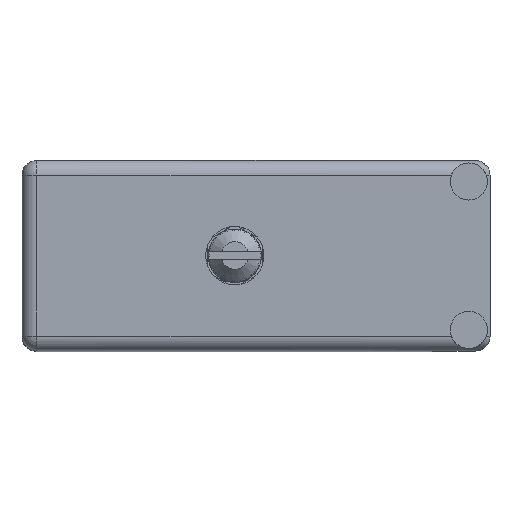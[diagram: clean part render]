
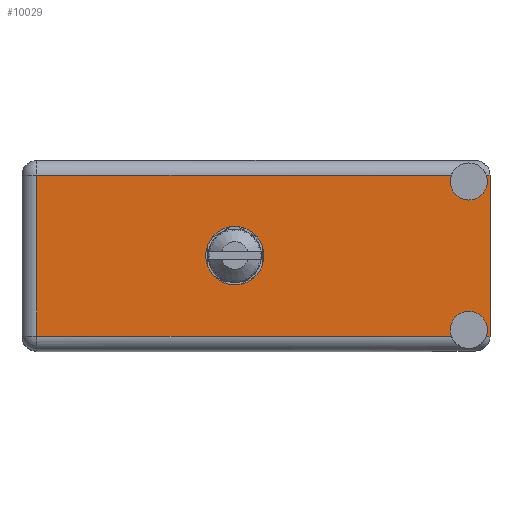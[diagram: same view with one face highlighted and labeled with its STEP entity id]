
A CAD part, top view. The second image highlights one B-rep face of the part: STEP entity #10029.
In plain terms, the highlighted face is planar.
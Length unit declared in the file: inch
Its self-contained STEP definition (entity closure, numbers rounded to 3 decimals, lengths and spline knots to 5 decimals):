
#2660 = EDGE_CURVE ( 'NONE', #68356, #49674, #86498, .T. ) ;
#3480 = DIRECTION ( 'NONE',  ( -1., 0., 0. ) ) ;
#7040 = AXIS2_PLACEMENT_3D ( 'NONE', #87515, #70118, #33771 ) ;
#8660 = ORIENTED_EDGE ( 'NONE', *, *, #97273, .F. ) ;
#10029 = ADVANCED_FACE ( 'NONE', ( #74525, #39920 ), #23921, .T. ) ;
#12254 = CARTESIAN_POINT ( 'NONE',  ( 1.204, 1.466, 0.3795 ) ) ;
#12378 = DIRECTION ( 'NONE',  ( 0., 0., 1. ) ) ;
#12601 = CARTESIAN_POINT ( 'NONE',  ( 1.18638, 1.466, 0.3795 ) ) ;
#12621 = ORIENTED_EDGE ( 'NONE', *, *, #48235, .T. ) ;
#12693 = VECTOR ( 'NONE', #94890, 39.37008 ) ;
#13507 = DIRECTION ( 'NONE',  ( 0., 1., 0. ) ) ;
#15020 = DIRECTION ( 'NONE',  ( 0., 1., 0. ) ) ;
#15229 = VECTOR ( 'NONE', #3480, 39.37008 ) ;
#16749 = ORIENTED_EDGE ( 'NONE', *, *, #27406, .F. ) ;
#18102 = CARTESIAN_POINT ( 'NONE',  ( 0., 1.466, 0. ) ) ;
#18825 = CARTESIAN_POINT ( 'NONE',  ( 1.204, 1.466, -0.3795 ) ) ;
#20325 = VECTOR ( 'NONE', #26297, 39.37008 ) ;
#23921 = PLANE ( 'NONE',  #24233 ) ;
#24233 = AXIS2_PLACEMENT_3D ( 'NONE', #24301, #15020, #112948 ) ;
#24301 = CARTESIAN_POINT ( 'NONE',  ( -1.004, 1.466, -0.4495 ) ) ;
#24703 = CIRCLE ( 'NONE', #62095, 0.1375 ) ;
#26297 = DIRECTION ( 'NONE',  ( -1., 0., 0. ) ) ;
#26575 = CARTESIAN_POINT ( 'NONE',  ( 1.104, 1.466, -0.2625 ) ) ;
#27406 = EDGE_CURVE ( 'NONE', #49674, #68356, #24703, .T. ) ;
#28528 = VECTOR ( 'NONE', #70282, 39.37008 ) ;
#30083 = AXIS2_PLACEMENT_3D ( 'NONE', #67349, #13507, #94017 ) ;
#31822 = ORIENTED_EDGE ( 'NONE', *, *, #79297, .T. ) ;
#32850 = VERTEX_POINT ( 'NONE', #46382 ) ;
#33526 = AXIS2_PLACEMENT_3D ( 'NONE', #114752, #53202, #61726 ) ;
#33771 = DIRECTION ( 'NONE',  ( 0., 0., 1. ) ) ;
#35325 = ORIENTED_EDGE ( 'NONE', *, *, #82789, .F. ) ;
#39052 = VERTEX_POINT ( 'NONE', #109235 ) ;
#39732 = CARTESIAN_POINT ( 'NONE',  ( 1.104, 1.466, 0.2625 ) ) ;
#39920 = FACE_OUTER_BOUND ( 'NONE', #98981, .T. ) ;
#40846 = VERTEX_POINT ( 'NONE', #26575 ) ;
#41012 = AXIS2_PLACEMENT_3D ( 'NONE', #105422, #43163, #105036 ) ;
#41634 = LINE ( 'NONE', #56622, #15229 ) ;
#43163 = DIRECTION ( 'NONE',  ( 0., 1., 0. ) ) ;
#43853 = CARTESIAN_POINT ( 'NONE',  ( 0., 1.466, 0.1375 ) ) ;
#44216 = EDGE_CURVE ( 'NONE', #54814, #94018, #106406, .T. ) ;
#45693 = EDGE_CURVE ( 'NONE', #59850, #95117, #46134, .T. ) ;
#46134 = CIRCLE ( 'NONE', #67799, 0.0875 ) ;
#46382 = CARTESIAN_POINT ( 'NONE',  ( 1.18638, 1.466, -0.3795 ) ) ;
#47016 = CARTESIAN_POINT ( 'NONE',  ( -0.934, 1.466, -0.3795 ) ) ;
#48092 = ORIENTED_EDGE ( 'NONE', *, *, #86106, .F. ) ;
#48235 = EDGE_CURVE ( 'NONE', #59850, #99988, #88930, .T. ) ;
#48389 = VECTOR ( 'NONE', #92002, 39.37008 ) ;
#49674 = VERTEX_POINT ( 'NONE', #92686 ) ;
#50212 = ORIENTED_EDGE ( 'NONE', *, *, #109368, .T. ) ;
#51059 = CARTESIAN_POINT ( 'NONE',  ( -0.934, 1.466, 0.3795 ) ) ;
#51062 = EDGE_CURVE ( 'NONE', #94018, #39052, #70531, .T. ) ;
#52126 = LINE ( 'NONE', #98083, #28528 ) ;
#53202 = DIRECTION ( 'NONE',  ( 0., 1., 0. ) ) ;
#54814 = VERTEX_POINT ( 'NONE', #47016 ) ;
#55426 = CIRCLE ( 'NONE', #33526, 0.0875 ) ;
#56526 = CARTESIAN_POINT ( 'NONE',  ( 1.104, 1.466, 0.35 ) ) ;
#56622 = CARTESIAN_POINT ( 'NONE',  ( -1.004, 1.466, -0.3795 ) ) ;
#56725 = VERTEX_POINT ( 'NONE', #111007 ) ;
#58659 = ORIENTED_EDGE ( 'NONE', *, *, #44216, .T. ) ;
#59850 = VERTEX_POINT ( 'NONE', #12601 ) ;
#61726 = DIRECTION ( 'NONE',  ( 0., 0., 1. ) ) ;
#61834 = ORIENTED_EDGE ( 'NONE', *, *, #2660, .F. ) ;
#61856 = DIRECTION ( 'NONE',  ( 0., 0., 1. ) ) ;
#62095 = AXIS2_PLACEMENT_3D ( 'NONE', #18102, #80007, #61856 ) ;
#64334 = VERTEX_POINT ( 'NONE', #18825 ) ;
#65453 = DIRECTION ( 'NONE',  ( 0., 1., 0. ) ) ;
#67349 = CARTESIAN_POINT ( 'NONE',  ( 1.104, 1.466, 0.35 ) ) ;
#67799 = AXIS2_PLACEMENT_3D ( 'NONE', #56526, #65453, #12378 ) ;
#68356 = VERTEX_POINT ( 'NONE', #43853 ) ;
#70118 = DIRECTION ( 'NONE',  ( 0., 1., 0. ) ) ;
#70282 = DIRECTION ( 'NONE',  ( 0., 0., 1. ) ) ;
#70531 = LINE ( 'NONE', #12254, #48389 ) ;
#71077 = ORIENTED_EDGE ( 'NONE', *, *, #90333, .F. ) ;
#71566 = CARTESIAN_POINT ( 'NONE',  ( -1.004, 1.466, -0.3795 ) ) ;
#72995 = LINE ( 'NONE', #71566, #20325 ) ;
#74092 = ORIENTED_EDGE ( 'NONE', *, *, #45693, .F. ) ;
#74525 = FACE_BOUND ( 'NONE', #97486, .T. ) ;
#79297 = EDGE_CURVE ( 'NONE', #56725, #54814, #41634, .T. ) ;
#80007 = DIRECTION ( 'NONE',  ( 0., 1., 0. ) ) ;
#82789 = EDGE_CURVE ( 'NONE', #64334, #99988, #52126, .T. ) ;
#83627 = CIRCLE ( 'NONE', #30083, 0.0875 ) ;
#86023 = CARTESIAN_POINT ( 'NONE',  ( 1.204, 1.466, 0.3795 ) ) ;
#86106 = EDGE_CURVE ( 'NONE', #95117, #39052, #83627, .T. ) ;
#86457 = CARTESIAN_POINT ( 'NONE',  ( 1.204, 1.466, 0.3795 ) ) ;
#86498 = CIRCLE ( 'NONE', #7040, 0.1375 ) ;
#87515 = CARTESIAN_POINT ( 'NONE',  ( 0., 1.466, 0. ) ) ;
#88930 = LINE ( 'NONE', #86023, #12693 ) ;
#90333 = EDGE_CURVE ( 'NONE', #56725, #40846, #55426, .T. ) ;
#91678 = CIRCLE ( 'NONE', #41012, 0.0875 ) ;
#92002 = DIRECTION ( 'NONE',  ( 1., 0., 0. ) ) ;
#92686 = CARTESIAN_POINT ( 'NONE',  ( 0., 1.466, -0.1375 ) ) ;
#93932 = VECTOR ( 'NONE', #96209, 39.37008 ) ;
#94017 = DIRECTION ( 'NONE',  ( 0., 0., 1. ) ) ;
#94018 = VERTEX_POINT ( 'NONE', #51059 ) ;
#94890 = DIRECTION ( 'NONE',  ( 1., 0., 0. ) ) ;
#95117 = VERTEX_POINT ( 'NONE', #39732 ) ;
#96209 = DIRECTION ( 'NONE',  ( 0., 0., 1. ) ) ;
#97273 = EDGE_CURVE ( 'NONE', #40846, #32850, #91678, .T. ) ;
#97486 = EDGE_LOOP ( 'NONE', ( #61834, #16749 ) ) ;
#98083 = CARTESIAN_POINT ( 'NONE',  ( 1.204, 1.466, 0.4495 ) ) ;
#98981 = EDGE_LOOP ( 'NONE', ( #113757, #48092, #74092, #12621, #35325, #50212, #8660, #71077, #31822, #58659 ) ) ;
#99988 = VERTEX_POINT ( 'NONE', #86457 ) ;
#105036 = DIRECTION ( 'NONE',  ( 0., 0., 1. ) ) ;
#105422 = CARTESIAN_POINT ( 'NONE',  ( 1.104, 1.466, -0.35 ) ) ;
#106406 = LINE ( 'NONE', #113256, #93932 ) ;
#109235 = CARTESIAN_POINT ( 'NONE',  ( 1.02162, 1.466, 0.3795 ) ) ;
#109368 = EDGE_CURVE ( 'NONE', #64334, #32850, #72995, .T. ) ;
#111007 = CARTESIAN_POINT ( 'NONE',  ( 1.02162, 1.466, -0.3795 ) ) ;
#112948 = DIRECTION ( 'NONE',  ( -1., 0., 0. ) ) ;
#113256 = CARTESIAN_POINT ( 'NONE',  ( -0.934, 1.466, -0.4495 ) ) ;
#113757 = ORIENTED_EDGE ( 'NONE', *, *, #51062, .T. ) ;
#114752 = CARTESIAN_POINT ( 'NONE',  ( 1.104, 1.466, -0.35 ) ) ;
